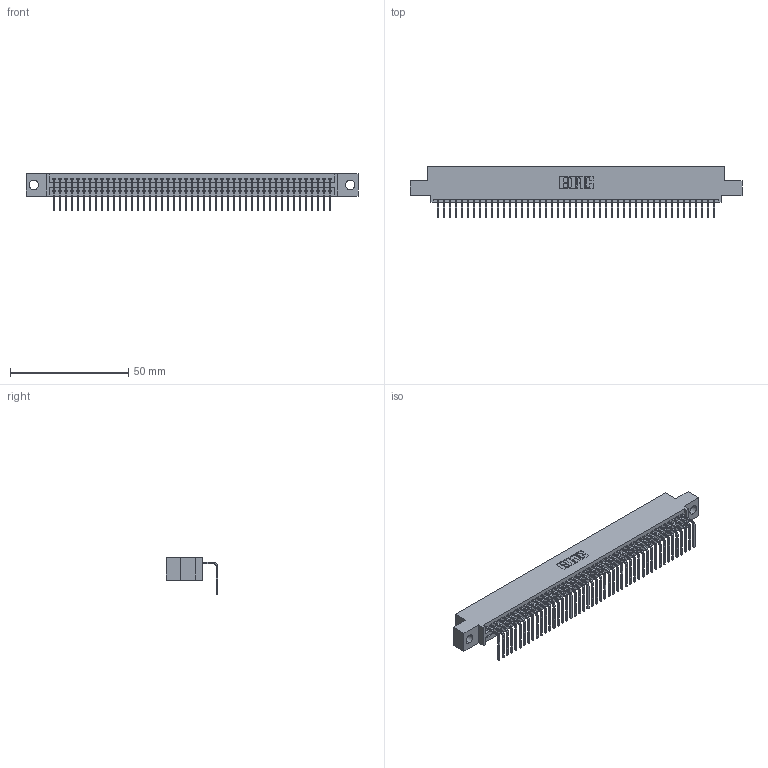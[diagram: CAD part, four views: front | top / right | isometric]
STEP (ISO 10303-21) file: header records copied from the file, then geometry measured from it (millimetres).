
FILE_DESCRIPTION (( 'STEP AP203' ), '1' );
FILE_NAME ('395-047-558-404.STEP', '2021-06-11T15:03:20', ( '' ), ( '' ), 'SwSTEP 2.0', 'SolidWorks 2020', '' );
FILE_SCHEMA (( 'CONFIG_CONTROL_DESIGN' ));
Length unit declared in the file: inch
Products named in the file (3): 345-292-001_558 Tail - 2; 395-047-558-404; 345 Part_0.110 Offset - 0.156 Dia-TI
Assembly tree (48 placements, depth 2):
  395-047-558-404
    345 Part_0.110 Offset - 0.156 Dia-TI
    345-292-001_558 Tail - 2  x47
Bounding box: 140.59 x 21.83 x 15.37 mm (x, y, z)
Volume: 13371.5 mm3; surface area: 18682 mm2
Topology: 48 solids, 48 shells, 2964 faces, 8943 edges, 5898 vertices
Faces by surface type: plane 2072, cylinder 892
Entity records: 35335 total; most frequent: CARTESIAN_POINT 6131, ORIENTED_EDGE 6110, DIRECTION 5345, EDGE_CURVE 3055, VECTOR 2735, LINE 2735, VERTEX_POINT 2034, AXIS2_PLACEMENT_3D 1305
